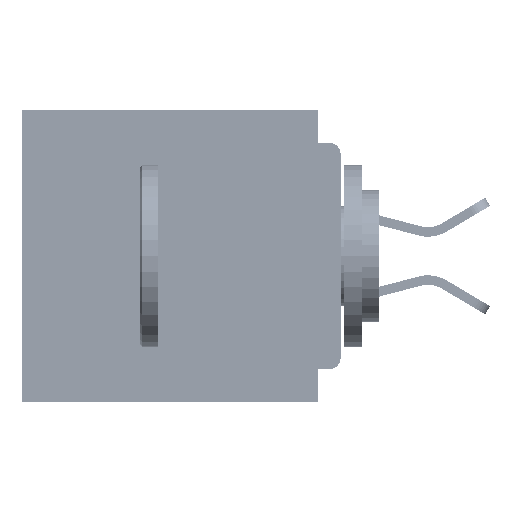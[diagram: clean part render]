
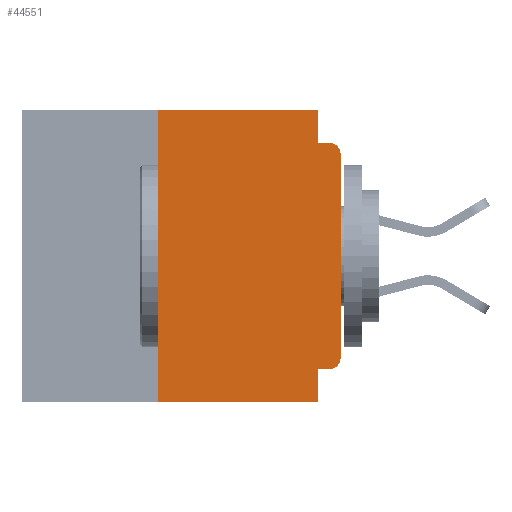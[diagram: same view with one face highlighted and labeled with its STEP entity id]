
A CAD part, left-side view. The second image highlights one B-rep face of the part: STEP entity #44551.
In plain terms, the highlighted planar face has unit normal (-1, 0, 0).
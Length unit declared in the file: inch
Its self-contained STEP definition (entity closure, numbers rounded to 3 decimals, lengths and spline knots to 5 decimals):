
#382 = DIRECTION ( 'NONE',  ( 0., -1., 0. ) ) ;
#1054 = EDGE_CURVE ( 'NONE', #38928, #2106, #29929, .T. ) ;
#1447 = LINE ( 'NONE', #15962, #42319 ) ;
#2106 = VERTEX_POINT ( 'NONE', #29238 ) ;
#2957 = CARTESIAN_POINT ( 'NONE',  ( 0., 0., -0.045 ) ) ;
#3966 = CARTESIAN_POINT ( 'NONE',  ( 0., 0.031, -0.355 ) ) ;
#4384 = EDGE_LOOP ( 'NONE', ( #22753, #46195, #51247, #43266, #29869, #41748, #43569, #14234, #28036, #23505 ) ) ;
#5355 = VECTOR ( 'NONE', #42476, 39.37008 ) ;
#5591 = EDGE_CURVE ( 'NONE', #12516, #38928, #41543, .T. ) ;
#6020 = LINE ( 'NONE', #49521, #24641 ) ;
#6407 = CARTESIAN_POINT ( 'NONE',  ( 0., 0.031, 0. ) ) ;
#7621 = VERTEX_POINT ( 'NONE', #3966 ) ;
#7730 = VERTEX_POINT ( 'NONE', #20658 ) ;
#8888 = VECTOR ( 'NONE', #382, 39.37008 ) ;
#9391 = LINE ( 'NONE', #40509, #50220 ) ;
#10418 = DIRECTION ( 'NONE',  ( 0., 0., -1. ) ) ;
#10775 = CARTESIAN_POINT ( 'NONE',  ( 0., 0.437, 0. ) ) ;
#10904 = CARTESIAN_POINT ( 'NONE',  ( 0., 0.25, 0. ) ) ;
#11236 = EDGE_CURVE ( 'NONE', #13553, #13577, #21177, .T. ) ;
#12516 = VERTEX_POINT ( 'NONE', #42015 ) ;
#12525 = CARTESIAN_POINT ( 'NONE',  ( 0., 0., -0.34 ) ) ;
#12793 = DIRECTION ( 'NONE',  ( -1., 0., 0. ) ) ;
#12794 = VECTOR ( 'NONE', #30614, 39.37008 ) ;
#13553 = VERTEX_POINT ( 'NONE', #44142 ) ;
#13577 = VERTEX_POINT ( 'NONE', #12525 ) ;
#14109 = VERTEX_POINT ( 'NONE', #47328 ) ;
#14234 = ORIENTED_EDGE ( 'NONE', *, *, #38764, .F. ) ;
#15962 = CARTESIAN_POINT ( 'NONE',  ( 0., 0., -0.355 ) ) ;
#17719 = DIRECTION ( 'NONE',  ( 0., 0., -1. ) ) ;
#18713 = CARTESIAN_POINT ( 'NONE',  ( 0., 0.015, -0.34 ) ) ;
#19116 = DIRECTION ( 'NONE',  ( 0., 0., -1. ) ) ;
#19287 = VECTOR ( 'NONE', #42509, 39.37008 ) ;
#19922 = DIRECTION ( 'NONE',  ( 0., 1., 0. ) ) ;
#20658 = CARTESIAN_POINT ( 'NONE',  ( 0., 0.015, -0.045 ) ) ;
#21177 = CIRCLE ( 'NONE', #28231, 0.015 ) ;
#21315 = VERTEX_POINT ( 'NONE', #50382 ) ;
#22696 = DIRECTION ( 'NONE',  ( 0., 0., -1. ) ) ;
#22753 = ORIENTED_EDGE ( 'NONE', *, *, #26142, .T. ) ;
#23505 = ORIENTED_EDGE ( 'NONE', *, *, #11236, .T. ) ;
#24641 = VECTOR ( 'NONE', #29822, 39.37008 ) ;
#26142 = EDGE_CURVE ( 'NONE', #13577, #21315, #35694, .T. ) ;
#27151 = AXIS2_PLACEMENT_3D ( 'NONE', #36445, #12793, #40448 ) ;
#27648 = VECTOR ( 'NONE', #10418, 39.37008 ) ;
#28036 = ORIENTED_EDGE ( 'NONE', *, *, #28648, .F. ) ;
#28231 = AXIS2_PLACEMENT_3D ( 'NONE', #18713, #46279, #22696 ) ;
#28648 = EDGE_CURVE ( 'NONE', #13553, #7621, #1447, .T. ) ;
#29238 = CARTESIAN_POINT ( 'NONE',  ( 0., 0.031, 0. ) ) ;
#29822 = DIRECTION ( 'NONE',  ( 0., -1., 0. ) ) ;
#29869 = ORIENTED_EDGE ( 'NONE', *, *, #1054, .F. ) ;
#29929 = LINE ( 'NONE', #42567, #8888 ) ;
#30072 = AXIS2_PLACEMENT_3D ( 'NONE', #10775, #42785, #19116 ) ;
#30614 = DIRECTION ( 'NONE',  ( 0., -1., 0. ) ) ;
#32691 = EDGE_CURVE ( 'NONE', #12516, #14109, #6020, .T. ) ;
#33313 = EDGE_CURVE ( 'NONE', #2106, #49748, #38125, .T. ) ;
#33875 = CIRCLE ( 'NONE', #27151, 0.015 ) ;
#35694 = LINE ( 'NONE', #38460, #5355 ) ;
#35763 = FACE_OUTER_BOUND ( 'NONE', #4384, .T. ) ;
#36445 = CARTESIAN_POINT ( 'NONE',  ( 0., 0.015, -0.06 ) ) ;
#38125 = LINE ( 'NONE', #6407, #27648 ) ;
#38233 = CARTESIAN_POINT ( 'NONE',  ( 0., 0.031, -0.045 ) ) ;
#38460 = CARTESIAN_POINT ( 'NONE',  ( 0., 0., 0. ) ) ;
#38764 = EDGE_CURVE ( 'NONE', #7621, #14109, #9391, .T. ) ;
#38765 = PLANE ( 'NONE',  #30072 ) ;
#38928 = VERTEX_POINT ( 'NONE', #10904 ) ;
#40448 = DIRECTION ( 'NONE',  ( 0., 0., -1. ) ) ;
#40509 = CARTESIAN_POINT ( 'NONE',  ( 0., 0.031, -0.4 ) ) ;
#41543 = LINE ( 'NONE', #42704, #19287 ) ;
#41748 = ORIENTED_EDGE ( 'NONE', *, *, #5591, .F. ) ;
#42015 = CARTESIAN_POINT ( 'NONE',  ( 0., 0.25, -0.4 ) ) ;
#42319 = VECTOR ( 'NONE', #19922, 39.37008 ) ;
#42476 = DIRECTION ( 'NONE',  ( 0., 0., 1. ) ) ;
#42509 = DIRECTION ( 'NONE',  ( 0., 0., 1. ) ) ;
#42567 = CARTESIAN_POINT ( 'NONE',  ( 0., 0.437, 0. ) ) ;
#42704 = CARTESIAN_POINT ( 'NONE',  ( 0., 0.25, -0.4 ) ) ;
#42785 = DIRECTION ( 'NONE',  ( 1., 0., 0. ) ) ;
#43086 = LINE ( 'NONE', #2957, #12794 ) ;
#43266 = ORIENTED_EDGE ( 'NONE', *, *, #33313, .F. ) ;
#43569 = ORIENTED_EDGE ( 'NONE', *, *, #32691, .T. ) ;
#44142 = CARTESIAN_POINT ( 'NONE',  ( 0., 0.015, -0.355 ) ) ;
#44551 = ADVANCED_FACE ( 'NONE', ( #35763 ), #38765, .F. ) ;
#45445 = EDGE_CURVE ( 'NONE', #21315, #7730, #33875, .T. ) ;
#46195 = ORIENTED_EDGE ( 'NONE', *, *, #45445, .T. ) ;
#46279 = DIRECTION ( 'NONE',  ( -1., 0., 0. ) ) ;
#46366 = EDGE_CURVE ( 'NONE', #49748, #7730, #43086, .T. ) ;
#47328 = CARTESIAN_POINT ( 'NONE',  ( 0., 0.031, -0.4 ) ) ;
#49521 = CARTESIAN_POINT ( 'NONE',  ( 0., 0.437, -0.4 ) ) ;
#49748 = VERTEX_POINT ( 'NONE', #38233 ) ;
#50220 = VECTOR ( 'NONE', #17719, 39.37008 ) ;
#50382 = CARTESIAN_POINT ( 'NONE',  ( 0., 0., -0.06 ) ) ;
#51247 = ORIENTED_EDGE ( 'NONE', *, *, #46366, .F. ) ;
